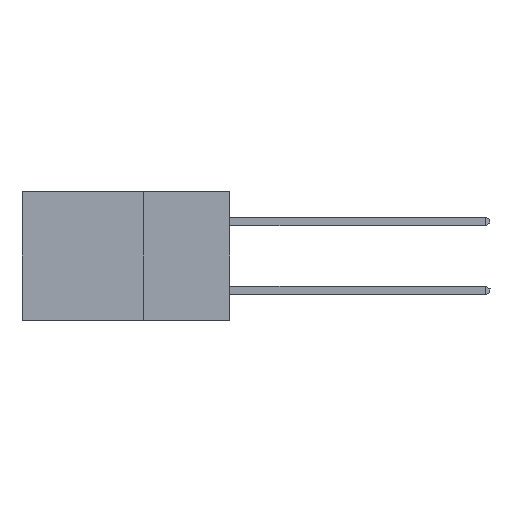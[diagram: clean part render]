
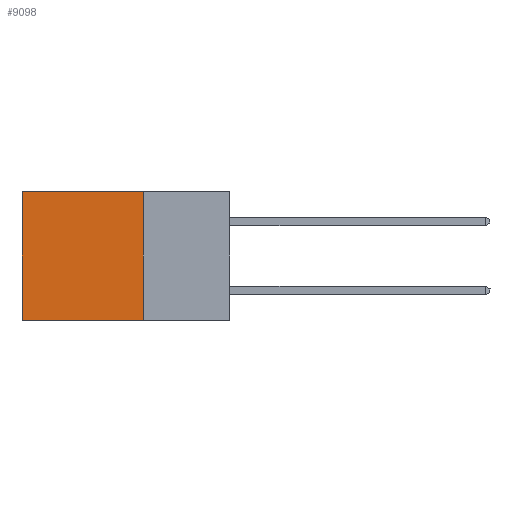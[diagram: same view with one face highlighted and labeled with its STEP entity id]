
A CAD part, left-side view. The second image highlights one B-rep face of the part: STEP entity #9098.
In plain terms, the highlighted planar face has unit normal (-1, 0, 0).
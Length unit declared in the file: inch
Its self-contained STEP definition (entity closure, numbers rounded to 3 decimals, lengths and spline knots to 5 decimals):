
#74 = PLANE ( 'NONE',  #23844 ) ;
#371 = CARTESIAN_POINT ( 'NONE',  ( 0.298, 0.6, 0. ) ) ;
#754 = CARTESIAN_POINT ( 'NONE',  ( 0.298, 0.25, -0.37 ) ) ;
#1155 = VERTEX_POINT ( 'NONE', #19581 ) ;
#2123 = DIRECTION ( 'NONE',  ( 0., 0., -1. ) ) ;
#2600 = EDGE_CURVE ( 'NONE', #23424, #13504, #15276, .T. ) ;
#2748 = LINE ( 'NONE', #25121, #5320 ) ;
#4565 = CARTESIAN_POINT ( 'NONE',  ( 0.298, 0.25, 0. ) ) ;
#5320 = VECTOR ( 'NONE', #24767, 39.37008 ) ;
#7016 = FACE_OUTER_BOUND ( 'NONE', #12083, .T. ) ;
#8686 = EDGE_CURVE ( 'NONE', #1155, #13504, #10237, .T. ) ;
#8734 = VERTEX_POINT ( 'NONE', #4565 ) ;
#9098 = ADVANCED_FACE ( 'NONE', ( #7016 ), #74, .F. ) ;
#9265 = VECTOR ( 'NONE', #24646, 39.37008 ) ;
#10237 = LINE ( 'NONE', #371, #9265 ) ;
#10413 = EDGE_CURVE ( 'NONE', #8734, #1155, #12731, .T. ) ;
#11849 = CARTESIAN_POINT ( 'NONE',  ( 0.298, 0.6, -0.37 ) ) ;
#12083 = EDGE_LOOP ( 'NONE', ( #15199, #16578, #19949, #26225 ) ) ;
#12731 = LINE ( 'NONE', #19822, #20814 ) ;
#13504 = VERTEX_POINT ( 'NONE', #11849 ) ;
#15199 = ORIENTED_EDGE ( 'NONE', *, *, #8686, .T. ) ;
#15276 = LINE ( 'NONE', #754, #20734 ) ;
#16116 = DIRECTION ( 'NONE',  ( 0., 1., 0. ) ) ;
#16343 = DIRECTION ( 'NONE',  ( 1., 0., 0. ) ) ;
#16578 = ORIENTED_EDGE ( 'NONE', *, *, #2600, .F. ) ;
#17484 = DIRECTION ( 'NONE',  ( 0., 1., 0. ) ) ;
#18957 = EDGE_CURVE ( 'NONE', #8734, #23424, #2748, .T. ) ;
#19581 = CARTESIAN_POINT ( 'NONE',  ( 0.298, 0.6, 0. ) ) ;
#19822 = CARTESIAN_POINT ( 'NONE',  ( 0.298, 0.25, 0. ) ) ;
#19949 = ORIENTED_EDGE ( 'NONE', *, *, #18957, .F. ) ;
#20734 = VECTOR ( 'NONE', #17484, 39.37008 ) ;
#20814 = VECTOR ( 'NONE', #16116, 39.37008 ) ;
#21544 = CARTESIAN_POINT ( 'NONE',  ( 0.298, 0.25, -0.37 ) ) ;
#22632 = CARTESIAN_POINT ( 'NONE',  ( 0.298, 0.25, 0. ) ) ;
#23424 = VERTEX_POINT ( 'NONE', #21544 ) ;
#23844 = AXIS2_PLACEMENT_3D ( 'NONE', #22632, #16343, #2123 ) ;
#24646 = DIRECTION ( 'NONE',  ( 0., 0., -1. ) ) ;
#24767 = DIRECTION ( 'NONE',  ( 0., 0., -1. ) ) ;
#25121 = CARTESIAN_POINT ( 'NONE',  ( 0.298, 0.25, 0. ) ) ;
#26225 = ORIENTED_EDGE ( 'NONE', *, *, #10413, .T. ) ;
